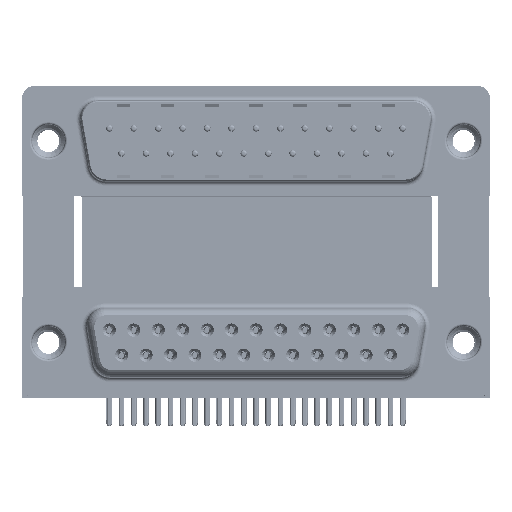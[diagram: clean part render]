
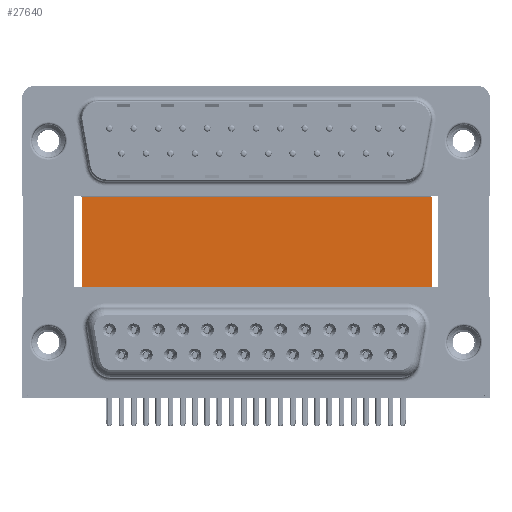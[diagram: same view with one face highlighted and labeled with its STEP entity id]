
A CAD part, top view. The second image highlights one B-rep face of the part: STEP entity #27640.
In plain terms, the highlighted planar face has unit normal (0, 0, 1).
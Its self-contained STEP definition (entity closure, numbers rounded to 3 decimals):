
#1498 = AXIS2_PLACEMENT_3D ( 'NONE', #46044, #4420, #21385 ) ;
#2171 = VECTOR ( 'NONE', #20918, 1000. ) ;
#3310 = CARTESIAN_POINT ( 'NONE',  ( 3.79, 16.585, -12. ) ) ;
#3882 = FACE_OUTER_BOUND ( 'NONE', #29002, .T. ) ;
#4420 = DIRECTION ( 'NONE',  ( 0., 0., -1. ) ) ;
#5567 = ORIENTED_EDGE ( 'NONE', *, *, #36958, .T. ) ;
#6612 = CARTESIAN_POINT ( 'NONE',  ( 3.79, 16.585, -12. ) ) ;
#7601 = VERTEX_POINT ( 'NONE', #32155 ) ;
#11030 = ORIENTED_EDGE ( 'NONE', *, *, #52912, .T. ) ;
#11234 = CARTESIAN_POINT ( 'NONE',  ( 43.43, 16.585, -12. ) ) ;
#16921 = VERTEX_POINT ( 'NONE', #11234 ) ;
#17219 = PLANE ( 'NONE',  #1498 ) ;
#19741 = DIRECTION ( 'NONE',  ( 0., -1., 0. ) ) ;
#20052 = VERTEX_POINT ( 'NONE', #34232 ) ;
#20918 = DIRECTION ( 'NONE',  ( 0., -1., 0. ) ) ;
#21112 = CARTESIAN_POINT ( 'NONE',  ( 3.79, -3.735, -12. ) ) ;
#21385 = DIRECTION ( 'NONE',  ( -1., 0., 0. ) ) ;
#23542 = DIRECTION ( 'NONE',  ( 1., 0., 0. ) ) ;
#24167 = ORIENTED_EDGE ( 'NONE', *, *, #37494, .F. ) ;
#27247 = VERTEX_POINT ( 'NONE', #27494 ) ;
#27260 = VECTOR ( 'NONE', #37726, 1000. ) ;
#27494 = CARTESIAN_POINT ( 'NONE',  ( 43.43, -3.735, -12. ) ) ;
#27640 = ADVANCED_FACE ( 'NONE', ( #3882 ), #17219, .F. ) ;
#27702 = LINE ( 'NONE', #6612, #43683 ) ;
#28737 = ORIENTED_EDGE ( 'NONE', *, *, #48152, .F. ) ;
#29002 = EDGE_LOOP ( 'NONE', ( #11030, #28737, #24167, #5567 ) ) ;
#32155 = CARTESIAN_POINT ( 'NONE',  ( 3.79, 16.585, -12. ) ) ;
#34232 = CARTESIAN_POINT ( 'NONE',  ( 3.79, -3.735, -12. ) ) ;
#36958 = EDGE_CURVE ( 'NONE', #7601, #20052, #49939, .T. ) ;
#37494 = EDGE_CURVE ( 'NONE', #7601, #16921, #27702, .T. ) ;
#37726 = DIRECTION ( 'NONE',  ( 1., 0., 0. ) ) ;
#37811 = LINE ( 'NONE', #38360, #2171 ) ;
#38360 = CARTESIAN_POINT ( 'NONE',  ( 43.43, 16.585, -12. ) ) ;
#38808 = LINE ( 'NONE', #21112, #27260 ) ;
#42718 = VECTOR ( 'NONE', #19741, 1000. ) ;
#43683 = VECTOR ( 'NONE', #23542, 1000. ) ;
#46044 = CARTESIAN_POINT ( 'NONE',  ( 3.79, 16.585, -12. ) ) ;
#48152 = EDGE_CURVE ( 'NONE', #16921, #27247, #37811, .T. ) ;
#49939 = LINE ( 'NONE', #3310, #42718 ) ;
#52912 = EDGE_CURVE ( 'NONE', #20052, #27247, #38808, .T. ) ;
